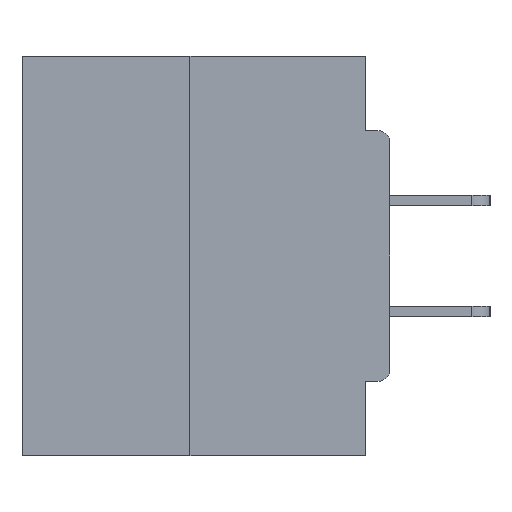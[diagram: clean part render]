
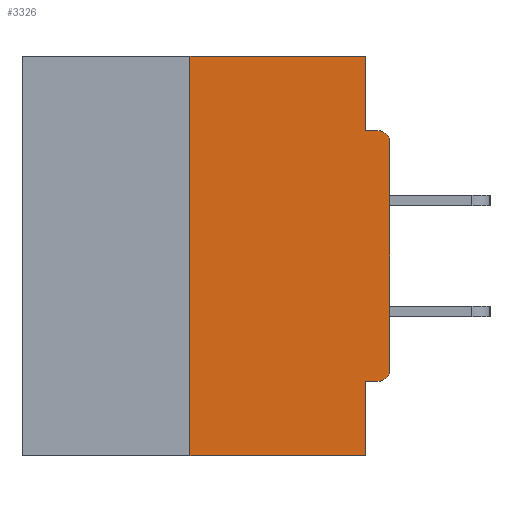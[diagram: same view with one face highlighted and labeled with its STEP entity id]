
A CAD part, left-side view. The second image highlights one B-rep face of the part: STEP entity #3326.
In plain terms, the highlighted planar face has unit normal (-1, 0, 0).
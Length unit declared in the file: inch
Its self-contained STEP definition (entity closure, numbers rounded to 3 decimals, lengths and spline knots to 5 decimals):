
#456 = ORIENTED_EDGE ( 'NONE', *, *, #23011, .T. ) ;
#1184 = CARTESIAN_POINT ( 'NONE',  ( 0., 0., -0.3915 ) ) ;
#1261 = ORIENTED_EDGE ( 'NONE', *, *, #19388, .T. ) ;
#1479 = CARTESIAN_POINT ( 'NONE',  ( 0., 0.015, -0.3915 ) ) ;
#1740 = DIRECTION ( 'NONE',  ( 0., -1., 0. ) ) ;
#1902 = LINE ( 'NONE', #17714, #32879 ) ;
#2152 = LINE ( 'NONE', #35171, #6203 ) ;
#2964 = LINE ( 'NONE', #19107, #29366 ) ;
#3326 = ADVANCED_FACE ( 'NONE', ( #36643 ), #8931, .F. ) ;
#3861 = VECTOR ( 'NONE', #9710, 39.37008 ) ;
#4645 = CARTESIAN_POINT ( 'NONE',  ( 0., 0.015, -0.0935 ) ) ;
#5134 = CARTESIAN_POINT ( 'NONE',  ( 0., 0.25, 0. ) ) ;
#5336 = AXIS2_PLACEMENT_3D ( 'NONE', #1479, #20321, #29617 ) ;
#6203 = VECTOR ( 'NONE', #25844, 39.37008 ) ;
#6633 = CIRCLE ( 'NONE', #5336, 0.015 ) ;
#7507 = ORIENTED_EDGE ( 'NONE', *, *, #17988, .T. ) ;
#7916 = DIRECTION ( 'NONE',  ( 0., 0., 1. ) ) ;
#8931 = PLANE ( 'NONE',  #22440 ) ;
#8937 = VERTEX_POINT ( 'NONE', #29379 ) ;
#9273 = EDGE_CURVE ( 'NONE', #38831, #21467, #25694, .T. ) ;
#9710 = DIRECTION ( 'NONE',  ( 0., 1., 0. ) ) ;
#10286 = AXIS2_PLACEMENT_3D ( 'NONE', #11778, #27955, #18456 ) ;
#10308 = CARTESIAN_POINT ( 'NONE',  ( 0., 0., -0.4065 ) ) ;
#11169 = CARTESIAN_POINT ( 'NONE',  ( 0., 0.46, 0. ) ) ;
#11359 = DIRECTION ( 'NONE',  ( 0., 0., -1. ) ) ;
#11778 = CARTESIAN_POINT ( 'NONE',  ( 0., 0.015, -0.1085 ) ) ;
#13959 = VERTEX_POINT ( 'NONE', #5134 ) ;
#14647 = CARTESIAN_POINT ( 'NONE',  ( 0., 0.25, 0. ) ) ;
#15000 = CARTESIAN_POINT ( 'NONE',  ( 0., 0.25, -0.5 ) ) ;
#15279 = EDGE_LOOP ( 'NONE', ( #19230, #15996, #1261, #29332, #27357, #7507, #456, #33006, #19127, #33134 ) ) ;
#15996 = ORIENTED_EDGE ( 'NONE', *, *, #39853, .F. ) ;
#16953 = CARTESIAN_POINT ( 'NONE',  ( 0., 0.46, 0. ) ) ;
#17207 = LINE ( 'NONE', #32773, #30959 ) ;
#17714 = CARTESIAN_POINT ( 'NONE',  ( 0., 0.031, -0.5 ) ) ;
#17988 = EDGE_CURVE ( 'NONE', #38831, #25094, #6633, .T. ) ;
#18456 = DIRECTION ( 'NONE',  ( 0., 0., -1. ) ) ;
#19107 = CARTESIAN_POINT ( 'NONE',  ( 0., 0., -0.0935 ) ) ;
#19127 = ORIENTED_EDGE ( 'NONE', *, *, #35546, .F. ) ;
#19230 = ORIENTED_EDGE ( 'NONE', *, *, #31872, .F. ) ;
#19306 = DIRECTION ( 'NONE',  ( 0., -1., 0. ) ) ;
#19388 = EDGE_CURVE ( 'NONE', #36250, #39502, #2152, .T. ) ;
#19420 = LINE ( 'NONE', #25285, #35937 ) ;
#20321 = DIRECTION ( 'NONE',  ( -1., 0., 0. ) ) ;
#21053 = VERTEX_POINT ( 'NONE', #28903 ) ;
#21134 = DIRECTION ( 'NONE',  ( 0., 0., -1. ) ) ;
#21467 = VERTEX_POINT ( 'NONE', #21982 ) ;
#21982 = CARTESIAN_POINT ( 'NONE',  ( 0., 0.031, -0.4065 ) ) ;
#22378 = EDGE_CURVE ( 'NONE', #21467, #39502, #1902, .T. ) ;
#22440 = AXIS2_PLACEMENT_3D ( 'NONE', #11169, #39102, #11359 ) ;
#22789 = EDGE_CURVE ( 'NONE', #21053, #39026, #31584, .T. ) ;
#23011 = EDGE_CURVE ( 'NONE', #25094, #21053, #17207, .T. ) ;
#25094 = VERTEX_POINT ( 'NONE', #1184 ) ;
#25095 = VERTEX_POINT ( 'NONE', #35612 ) ;
#25285 = CARTESIAN_POINT ( 'NONE',  ( 0., 0.031, 0. ) ) ;
#25694 = LINE ( 'NONE', #10308, #3861 ) ;
#25844 = DIRECTION ( 'NONE',  ( 0., -1., 0. ) ) ;
#26005 = VECTOR ( 'NONE', #1740, 39.37008 ) ;
#27357 = ORIENTED_EDGE ( 'NONE', *, *, #9273, .F. ) ;
#27604 = VECTOR ( 'NONE', #39734, 39.37008 ) ;
#27955 = DIRECTION ( 'NONE',  ( -1., 0., 0. ) ) ;
#28903 = CARTESIAN_POINT ( 'NONE',  ( 0., 0., -0.1085 ) ) ;
#29131 = CARTESIAN_POINT ( 'NONE',  ( 0., 0.015, -0.4065 ) ) ;
#29332 = ORIENTED_EDGE ( 'NONE', *, *, #22378, .F. ) ;
#29366 = VECTOR ( 'NONE', #19306, 39.37008 ) ;
#29379 = CARTESIAN_POINT ( 'NONE',  ( 0., 0.031, 0. ) ) ;
#29617 = DIRECTION ( 'NONE',  ( 0., 0., -1. ) ) ;
#29692 = LINE ( 'NONE', #16953, #26005 ) ;
#30515 = EDGE_CURVE ( 'NONE', #8937, #25095, #19420, .T. ) ;
#30658 = CARTESIAN_POINT ( 'NONE',  ( 0., 0.031, -0.5 ) ) ;
#30959 = VECTOR ( 'NONE', #7916, 39.37008 ) ;
#31584 = CIRCLE ( 'NONE', #10286, 0.015 ) ;
#31872 = EDGE_CURVE ( 'NONE', #13959, #8937, #29692, .T. ) ;
#32773 = CARTESIAN_POINT ( 'NONE',  ( 0., 0., 0. ) ) ;
#32879 = VECTOR ( 'NONE', #21134, 39.37008 ) ;
#33006 = ORIENTED_EDGE ( 'NONE', *, *, #22789, .T. ) ;
#33134 = ORIENTED_EDGE ( 'NONE', *, *, #30515, .F. ) ;
#33649 = LINE ( 'NONE', #14647, #27604 ) ;
#35171 = CARTESIAN_POINT ( 'NONE',  ( 0., 0.46, -0.5 ) ) ;
#35546 = EDGE_CURVE ( 'NONE', #25095, #39026, #2964, .T. ) ;
#35612 = CARTESIAN_POINT ( 'NONE',  ( 0., 0.031, -0.0935 ) ) ;
#35937 = VECTOR ( 'NONE', #37638, 39.37008 ) ;
#36250 = VERTEX_POINT ( 'NONE', #15000 ) ;
#36643 = FACE_OUTER_BOUND ( 'NONE', #15279, .T. ) ;
#37638 = DIRECTION ( 'NONE',  ( 0., 0., -1. ) ) ;
#38831 = VERTEX_POINT ( 'NONE', #29131 ) ;
#39026 = VERTEX_POINT ( 'NONE', #4645 ) ;
#39102 = DIRECTION ( 'NONE',  ( 1., 0., 0. ) ) ;
#39502 = VERTEX_POINT ( 'NONE', #30658 ) ;
#39734 = DIRECTION ( 'NONE',  ( 0., 0., 1. ) ) ;
#39853 = EDGE_CURVE ( 'NONE', #36250, #13959, #33649, .T. ) ;
